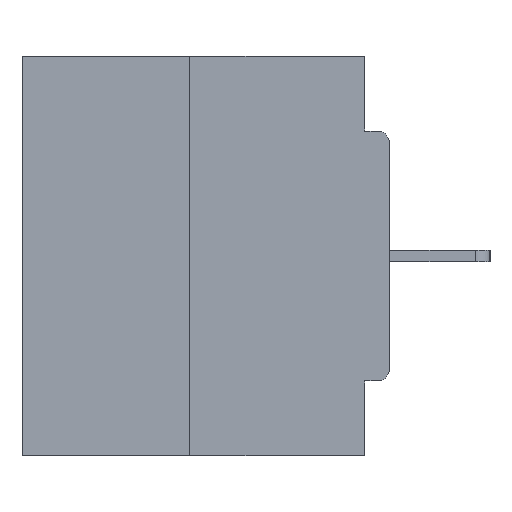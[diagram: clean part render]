
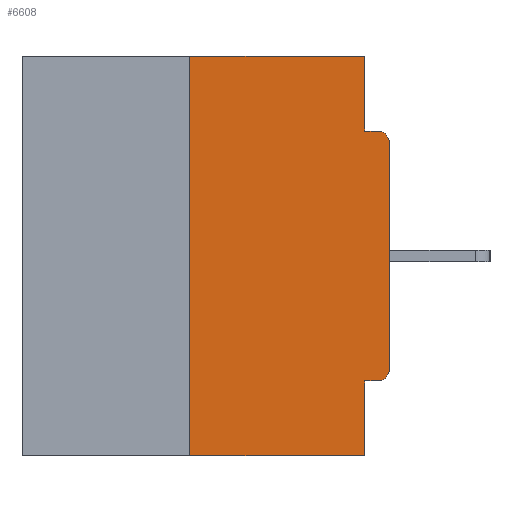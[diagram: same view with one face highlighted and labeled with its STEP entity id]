
A CAD part, left-side view. The second image highlights one B-rep face of the part: STEP entity #6608.
In plain terms, the highlighted planar face has unit normal (-1, 0, 0).
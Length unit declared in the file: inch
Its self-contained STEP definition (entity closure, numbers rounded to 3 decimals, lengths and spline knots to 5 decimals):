
#353 = VECTOR ( 'NONE', #38099, 39.37008 ) ;
#433 = CIRCLE ( 'NONE', #12788, 0.015 ) ;
#783 = DIRECTION ( 'NONE',  ( -1., 0., 0. ) ) ;
#1047 = DIRECTION ( 'NONE',  ( 0., -1., 0. ) ) ;
#1812 = ORIENTED_EDGE ( 'NONE', *, *, #32989, .T. ) ;
#1881 = EDGE_CURVE ( 'NONE', #11999, #32376, #20412, .T. ) ;
#1898 = LINE ( 'NONE', #17190, #3444 ) ;
#2007 = ORIENTED_EDGE ( 'NONE', *, *, #18206, .F. ) ;
#2230 = PLANE ( 'NONE',  #31297 ) ;
#2710 = VERTEX_POINT ( 'NONE', #8901 ) ;
#3303 = CARTESIAN_POINT ( 'NONE',  ( 0., 0.031, -0.4065 ) ) ;
#3444 = VECTOR ( 'NONE', #28998, 39.37008 ) ;
#3678 = VERTEX_POINT ( 'NONE', #7586 ) ;
#3700 = CARTESIAN_POINT ( 'NONE',  ( 0., 0.46, -0.5 ) ) ;
#3968 = VECTOR ( 'NONE', #9277, 39.37008 ) ;
#3977 = CARTESIAN_POINT ( 'NONE',  ( 0., 0.015, -0.0935 ) ) ;
#4799 = VERTEX_POINT ( 'NONE', #32969 ) ;
#4823 = CARTESIAN_POINT ( 'NONE',  ( 0., 0., -0.0935 ) ) ;
#4872 = CARTESIAN_POINT ( 'NONE',  ( 0., 0., -0.1085 ) ) ;
#6189 = EDGE_CURVE ( 'NONE', #2710, #17834, #11554, .T. ) ;
#6410 = EDGE_CURVE ( 'NONE', #9733, #11999, #27609, .T. ) ;
#6608 = ADVANCED_FACE ( 'NONE', ( #25639 ), #2230, .F. ) ;
#7586 = CARTESIAN_POINT ( 'NONE',  ( 0., 0.031, 0. ) ) ;
#7720 = LINE ( 'NONE', #4823, #31059 ) ;
#8901 = CARTESIAN_POINT ( 'NONE',  ( 0., 0., -0.3915 ) ) ;
#9277 = DIRECTION ( 'NONE',  ( 0., 0., -1. ) ) ;
#9733 = VERTEX_POINT ( 'NONE', #15926 ) ;
#10448 = CIRCLE ( 'NONE', #20339, 0.015 ) ;
#11146 = CARTESIAN_POINT ( 'NONE',  ( 0., 0.46, 0. ) ) ;
#11295 = CARTESIAN_POINT ( 'NONE',  ( 0., 0.031, -0.5 ) ) ;
#11554 = LINE ( 'NONE', #26647, #353 ) ;
#11991 = VERTEX_POINT ( 'NONE', #29249 ) ;
#11998 = EDGE_CURVE ( 'NONE', #11991, #32376, #12222, .T. ) ;
#11999 = VERTEX_POINT ( 'NONE', #3303 ) ;
#12052 = DIRECTION ( 'NONE',  ( 0., 0., -1. ) ) ;
#12222 = LINE ( 'NONE', #3700, #37348 ) ;
#12239 = CARTESIAN_POINT ( 'NONE',  ( 0., 0.015, -0.3915 ) ) ;
#12462 = EDGE_CURVE ( 'NONE', #3678, #32238, #35827, .T. ) ;
#12788 = AXIS2_PLACEMENT_3D ( 'NONE', #12239, #783, #15341 ) ;
#13317 = CARTESIAN_POINT ( 'NONE',  ( 0., 0.015, -0.1085 ) ) ;
#14034 = DIRECTION ( 'NONE',  ( 1., 0., 0. ) ) ;
#15341 = DIRECTION ( 'NONE',  ( 0., 0., -1. ) ) ;
#15626 = VERTEX_POINT ( 'NONE', #3977 ) ;
#15926 = CARTESIAN_POINT ( 'NONE',  ( 0., 0.015, -0.4065 ) ) ;
#16190 = ORIENTED_EDGE ( 'NONE', *, *, #12462, .F. ) ;
#16212 = ORIENTED_EDGE ( 'NONE', *, *, #11998, .T. ) ;
#17190 = CARTESIAN_POINT ( 'NONE',  ( 0., 0.25, 0. ) ) ;
#17272 = EDGE_CURVE ( 'NONE', #4799, #3678, #30464, .T. ) ;
#17834 = VERTEX_POINT ( 'NONE', #4872 ) ;
#18206 = EDGE_CURVE ( 'NONE', #11991, #4799, #1898, .T. ) ;
#18219 = DIRECTION ( 'NONE',  ( 0., -1., 0. ) ) ;
#18692 = CARTESIAN_POINT ( 'NONE',  ( 0., 0., -0.4065 ) ) ;
#20339 = AXIS2_PLACEMENT_3D ( 'NONE', #13317, #36967, #30553 ) ;
#20412 = LINE ( 'NONE', #11295, #38295 ) ;
#20499 = CARTESIAN_POINT ( 'NONE',  ( 0., 0.031, 0. ) ) ;
#21735 = ORIENTED_EDGE ( 'NONE', *, *, #1881, .F. ) ;
#23743 = EDGE_CURVE ( 'NONE', #9733, #2710, #433, .T. ) ;
#25512 = DIRECTION ( 'NONE',  ( 0., -1., 0. ) ) ;
#25639 = FACE_OUTER_BOUND ( 'NONE', #26928, .T. ) ;
#25844 = DIRECTION ( 'NONE',  ( 0., 0., -1. ) ) ;
#26036 = CARTESIAN_POINT ( 'NONE',  ( 0., 0.031, -0.0935 ) ) ;
#26246 = VECTOR ( 'NONE', #1047, 39.37008 ) ;
#26647 = CARTESIAN_POINT ( 'NONE',  ( 0., 0., 0. ) ) ;
#26928 = EDGE_LOOP ( 'NONE', ( #30390, #2007, #16212, #21735, #30894, #35917, #36077, #1812, #38280, #16190 ) ) ;
#27609 = LINE ( 'NONE', #18692, #28268 ) ;
#27812 = DIRECTION ( 'NONE',  ( 0., 1., 0. ) ) ;
#28268 = VECTOR ( 'NONE', #27812, 39.37008 ) ;
#28998 = DIRECTION ( 'NONE',  ( 0., 0., 1. ) ) ;
#29249 = CARTESIAN_POINT ( 'NONE',  ( 0., 0.25, -0.5 ) ) ;
#30390 = ORIENTED_EDGE ( 'NONE', *, *, #17272, .F. ) ;
#30464 = LINE ( 'NONE', #33568, #26246 ) ;
#30553 = DIRECTION ( 'NONE',  ( 0., 0., -1. ) ) ;
#30894 = ORIENTED_EDGE ( 'NONE', *, *, #6410, .F. ) ;
#31059 = VECTOR ( 'NONE', #25512, 39.37008 ) ;
#31297 = AXIS2_PLACEMENT_3D ( 'NONE', #11146, #14034, #25844 ) ;
#32238 = VERTEX_POINT ( 'NONE', #26036 ) ;
#32376 = VERTEX_POINT ( 'NONE', #36458 ) ;
#32969 = CARTESIAN_POINT ( 'NONE',  ( 0., 0.25, 0. ) ) ;
#32989 = EDGE_CURVE ( 'NONE', #17834, #15626, #10448, .T. ) ;
#33568 = CARTESIAN_POINT ( 'NONE',  ( 0., 0.46, 0. ) ) ;
#35827 = LINE ( 'NONE', #20499, #3968 ) ;
#35909 = EDGE_CURVE ( 'NONE', #32238, #15626, #7720, .T. ) ;
#35917 = ORIENTED_EDGE ( 'NONE', *, *, #23743, .T. ) ;
#36077 = ORIENTED_EDGE ( 'NONE', *, *, #6189, .T. ) ;
#36458 = CARTESIAN_POINT ( 'NONE',  ( 0., 0.031, -0.5 ) ) ;
#36967 = DIRECTION ( 'NONE',  ( -1., 0., 0. ) ) ;
#37348 = VECTOR ( 'NONE', #18219, 39.37008 ) ;
#38099 = DIRECTION ( 'NONE',  ( 0., 0., 1. ) ) ;
#38280 = ORIENTED_EDGE ( 'NONE', *, *, #35909, .F. ) ;
#38295 = VECTOR ( 'NONE', #12052, 39.37008 ) ;
